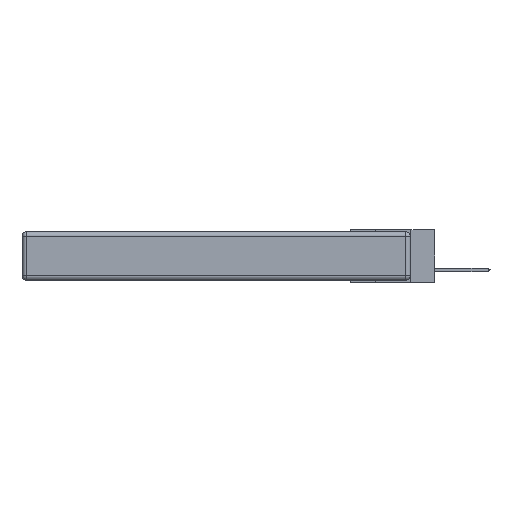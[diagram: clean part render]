
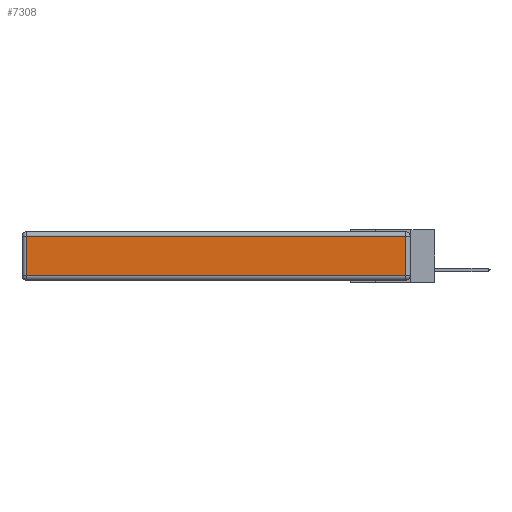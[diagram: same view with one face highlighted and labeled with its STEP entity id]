
A CAD part, left-side view. The second image highlights one B-rep face of the part: STEP entity #7308.
In plain terms, the highlighted planar face has unit normal (-1, 0, 0).
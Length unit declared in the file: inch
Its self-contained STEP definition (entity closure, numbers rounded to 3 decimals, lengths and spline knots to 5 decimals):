
#1930 = DIRECTION ( 'NONE',  ( 0., 0., -1. ) ) ;
#2321 = VERTEX_POINT ( 'NONE', #8979 ) ;
#2369 = EDGE_CURVE ( 'NONE', #8109, #2321, #19161, .T. ) ;
#2521 = EDGE_LOOP ( 'NONE', ( #7691, #20159, #11392, #3158 ) ) ;
#3158 = ORIENTED_EDGE ( 'NONE', *, *, #21478, .T. ) ;
#5328 = FACE_OUTER_BOUND ( 'NONE', #2521, .T. ) ;
#5691 = DIRECTION ( 'NONE',  ( 0., -1., 0. ) ) ;
#6521 = LINE ( 'NONE', #18573, #25268 ) ;
#6901 = CARTESIAN_POINT ( 'NONE',  ( 0., 0.03, -0.343 ) ) ;
#7308 = ADVANCED_FACE ( 'NONE', ( #5328 ), #14586, .T. ) ;
#7586 = VERTEX_POINT ( 'NONE', #19452 ) ;
#7691 = ORIENTED_EDGE ( 'NONE', *, *, #16340, .T. ) ;
#8109 = VERTEX_POINT ( 'NONE', #25656 ) ;
#8979 = CARTESIAN_POINT ( 'NONE',  ( 0., 0.03, -0.03 ) ) ;
#9287 = CARTESIAN_POINT ( 'NONE',  ( 0., 2.72, -0.03 ) ) ;
#10185 = VECTOR ( 'NONE', #5691, 39.37008 ) ;
#10317 = CARTESIAN_POINT ( 'NONE',  ( 0., 0., -0.343 ) ) ;
#10507 = LINE ( 'NONE', #20179, #10185 ) ;
#11392 = ORIENTED_EDGE ( 'NONE', *, *, #14539, .T. ) ;
#11874 = AXIS2_PLACEMENT_3D ( 'NONE', #10317, #24761, #14494 ) ;
#12691 = VECTOR ( 'NONE', #13145, 39.37008 ) ;
#13145 = DIRECTION ( 'NONE',  ( 0., 0., 1. ) ) ;
#13757 = DIRECTION ( 'NONE',  ( 0., 1., 0. ) ) ;
#14099 = CARTESIAN_POINT ( 'NONE',  ( 0., 2.75, -0.03 ) ) ;
#14494 = DIRECTION ( 'NONE',  ( 0., 0., 1. ) ) ;
#14539 = EDGE_CURVE ( 'NONE', #2321, #25683, #17469, .T. ) ;
#14586 = PLANE ( 'NONE',  #11874 ) ;
#16340 = EDGE_CURVE ( 'NONE', #7586, #8109, #10507, .T. ) ;
#16455 = VECTOR ( 'NONE', #13757, 39.37008 ) ;
#17469 = LINE ( 'NONE', #14099, #16455 ) ;
#18573 = CARTESIAN_POINT ( 'NONE',  ( 0., 2.72, -0.343 ) ) ;
#19161 = LINE ( 'NONE', #6901, #12691 ) ;
#19452 = CARTESIAN_POINT ( 'NONE',  ( 0., 2.72, -0.313 ) ) ;
#20159 = ORIENTED_EDGE ( 'NONE', *, *, #2369, .T. ) ;
#20179 = CARTESIAN_POINT ( 'NONE',  ( 0., 0., -0.313 ) ) ;
#21478 = EDGE_CURVE ( 'NONE', #25683, #7586, #6521, .T. ) ;
#24761 = DIRECTION ( 'NONE',  ( -1., 0., 0. ) ) ;
#25268 = VECTOR ( 'NONE', #1930, 39.37008 ) ;
#25656 = CARTESIAN_POINT ( 'NONE',  ( 0., 0.03, -0.313 ) ) ;
#25683 = VERTEX_POINT ( 'NONE', #9287 ) ;
